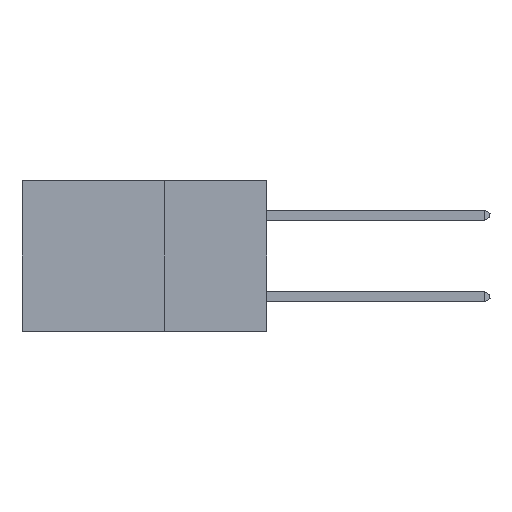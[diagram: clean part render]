
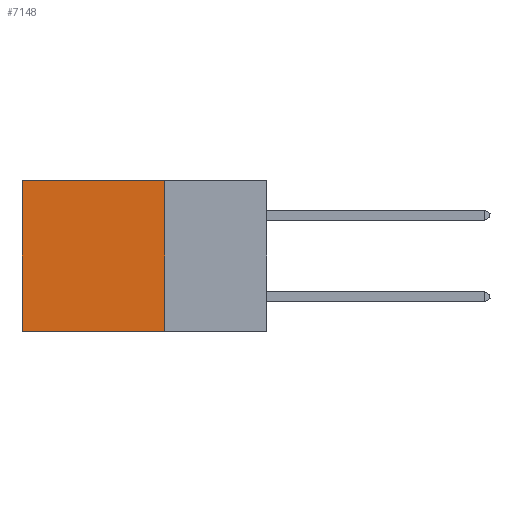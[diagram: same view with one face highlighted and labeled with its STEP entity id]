
A CAD part, left-side view. The second image highlights one B-rep face of the part: STEP entity #7148.
In plain terms, the highlighted planar face has unit normal (-1, 0, 0).
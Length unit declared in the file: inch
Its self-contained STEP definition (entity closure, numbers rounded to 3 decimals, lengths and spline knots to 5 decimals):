
#557 = EDGE_CURVE ( 'NONE', #6962, #24106, #16631, .T. ) ;
#740 = DIRECTION ( 'NONE',  ( 0., 0., -1. ) ) ;
#1334 = FACE_OUTER_BOUND ( 'NONE', #19501, .T. ) ;
#2570 = PLANE ( 'NONE',  #15297 ) ;
#2573 = CARTESIAN_POINT ( 'NONE',  ( 0.2875, 0.25, 0. ) ) ;
#2670 = ORIENTED_EDGE ( 'NONE', *, *, #18479, .F. ) ;
#4638 = VECTOR ( 'NONE', #6683, 39.37008 ) ;
#6683 = DIRECTION ( 'NONE',  ( 0., 0., -1. ) ) ;
#6962 = VERTEX_POINT ( 'NONE', #22588 ) ;
#7097 = DIRECTION ( 'NONE',  ( 0., 1., 0. ) ) ;
#7148 = ADVANCED_FACE ( 'NONE', ( #1334 ), #2570, .F. ) ;
#8934 = DIRECTION ( 'NONE',  ( 0., 1., 0. ) ) ;
#9993 = LINE ( 'NONE', #21989, #17392 ) ;
#10438 = ORIENTED_EDGE ( 'NONE', *, *, #557, .T. ) ;
#10981 = CARTESIAN_POINT ( 'NONE',  ( 0.2875, 0.25, 0. ) ) ;
#11224 = VERTEX_POINT ( 'NONE', #2573 ) ;
#12166 = CARTESIAN_POINT ( 'NONE',  ( 0.2875, 0.25, 0. ) ) ;
#12210 = VECTOR ( 'NONE', #18294, 39.37008 ) ;
#13242 = LINE ( 'NONE', #10981, #18545 ) ;
#14326 = VERTEX_POINT ( 'NONE', #21740 ) ;
#15274 = ORIENTED_EDGE ( 'NONE', *, *, #18371, .F. ) ;
#15297 = AXIS2_PLACEMENT_3D ( 'NONE', #12166, #19742, #740 ) ;
#16631 = LINE ( 'NONE', #24060, #12210 ) ;
#17392 = VECTOR ( 'NONE', #8934, 39.37008 ) ;
#17731 = ORIENTED_EDGE ( 'NONE', *, *, #19212, .T. ) ;
#18045 = CARTESIAN_POINT ( 'NONE',  ( 0.2875, 0.25, 0. ) ) ;
#18294 = DIRECTION ( 'NONE',  ( 0., 0., -1. ) ) ;
#18371 = EDGE_CURVE ( 'NONE', #11224, #14326, #23885, .T. ) ;
#18479 = EDGE_CURVE ( 'NONE', #14326, #24106, #9993, .T. ) ;
#18545 = VECTOR ( 'NONE', #7097, 39.37008 ) ;
#19212 = EDGE_CURVE ( 'NONE', #11224, #6962, #13242, .T. ) ;
#19372 = CARTESIAN_POINT ( 'NONE',  ( 0.2875, 0.6, -0.37 ) ) ;
#19501 = EDGE_LOOP ( 'NONE', ( #10438, #2670, #15274, #17731 ) ) ;
#19742 = DIRECTION ( 'NONE',  ( 1., 0., 0. ) ) ;
#21740 = CARTESIAN_POINT ( 'NONE',  ( 0.2875, 0.25, -0.37 ) ) ;
#21989 = CARTESIAN_POINT ( 'NONE',  ( 0.2875, 0.25, -0.37 ) ) ;
#22588 = CARTESIAN_POINT ( 'NONE',  ( 0.2875, 0.6, 0. ) ) ;
#23885 = LINE ( 'NONE', #18045, #4638 ) ;
#24060 = CARTESIAN_POINT ( 'NONE',  ( 0.2875, 0.6, 0. ) ) ;
#24106 = VERTEX_POINT ( 'NONE', #19372 ) ;
